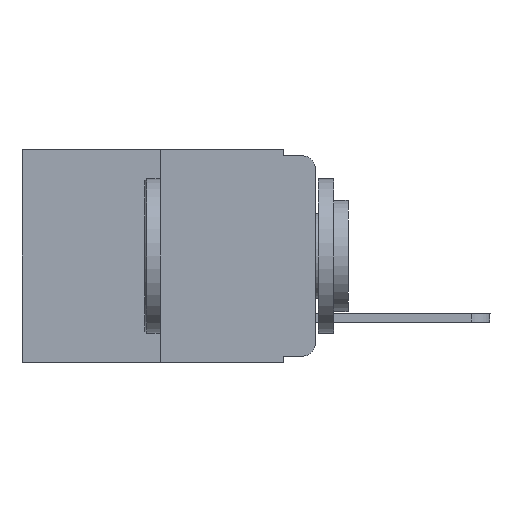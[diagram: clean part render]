
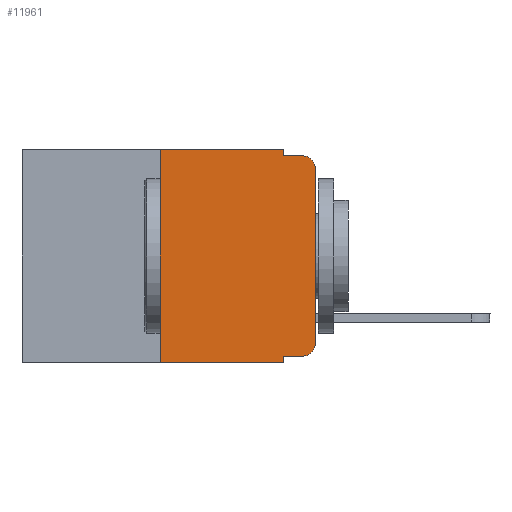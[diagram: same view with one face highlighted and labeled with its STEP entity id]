
A CAD part, left-side view. The second image highlights one B-rep face of the part: STEP entity #11961.
In plain terms, the highlighted planar face has unit normal (-1, 0, 0).
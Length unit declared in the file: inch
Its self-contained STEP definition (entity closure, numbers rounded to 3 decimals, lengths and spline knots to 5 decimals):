
#108 = CARTESIAN_POINT ( 'NONE',  ( 0., 0.02, -0.03 ) ) ;
#136 = DIRECTION ( 'NONE',  ( 0., 0., 1. ) ) ;
#485 = EDGE_CURVE ( 'NONE', #8665, #13076, #2736, .T. ) ;
#752 = VECTOR ( 'NONE', #2360, 39.37008 ) ;
#754 = ORIENTED_EDGE ( 'NONE', *, *, #22057, .T. ) ;
#1009 = DIRECTION ( 'NONE',  ( -1., 0., 0. ) ) ;
#1392 = CIRCLE ( 'NONE', #2554, 0.02 ) ;
#1819 = EDGE_CURVE ( 'NONE', #18879, #10111, #19831, .T. ) ;
#2360 = DIRECTION ( 'NONE',  ( 0., 0., -1. ) ) ;
#2554 = AXIS2_PLACEMENT_3D ( 'NONE', #108, #14737, #12557 ) ;
#2681 = CARTESIAN_POINT ( 'NONE',  ( 0., 0.473, 0. ) ) ;
#2736 = CIRCLE ( 'NONE', #9696, 0.02 ) ;
#2894 = DIRECTION ( 'NONE',  ( 0., -1., 0. ) ) ;
#3457 = ORIENTED_EDGE ( 'NONE', *, *, #5356, .F. ) ;
#3514 = VERTEX_POINT ( 'NONE', #14133 ) ;
#3524 = LINE ( 'NONE', #22312, #7562 ) ;
#3659 = VECTOR ( 'NONE', #22688, 39.37008 ) ;
#3945 = LINE ( 'NONE', #9612, #752 ) ;
#3981 = LINE ( 'NONE', #17259, #8720 ) ;
#4107 = VERTEX_POINT ( 'NONE', #16876 ) ;
#4169 = ORIENTED_EDGE ( 'NONE', *, *, #1819, .F. ) ;
#5329 = DIRECTION ( 'NONE',  ( 1., 0., 0. ) ) ;
#5356 = EDGE_CURVE ( 'NONE', #3514, #12157, #3945, .T. ) ;
#5535 = EDGE_CURVE ( 'NONE', #13076, #16201, #22835, .T. ) ;
#5850 = VECTOR ( 'NONE', #2894, 39.37008 ) ;
#6063 = VECTOR ( 'NONE', #17531, 39.37008 ) ;
#6206 = EDGE_CURVE ( 'NONE', #23818, #17589, #3524, .T. ) ;
#6356 = ORIENTED_EDGE ( 'NONE', *, *, #6206, .F. ) ;
#6937 = DIRECTION ( 'NONE',  ( 0., 0., -1. ) ) ;
#7132 = ORIENTED_EDGE ( 'NONE', *, *, #15528, .F. ) ;
#7562 = VECTOR ( 'NONE', #136, 39.37008 ) ;
#7708 = CARTESIAN_POINT ( 'NONE',  ( 0., 0., -0.03 ) ) ;
#7861 = CARTESIAN_POINT ( 'NONE',  ( 0., 0.051, -0.343 ) ) ;
#8154 = CARTESIAN_POINT ( 'NONE',  ( 0., 0., 0. ) ) ;
#8665 = VERTEX_POINT ( 'NONE', #22729 ) ;
#8720 = VECTOR ( 'NONE', #22639, 39.37008 ) ;
#8829 = FACE_OUTER_BOUND ( 'NONE', #22675, .T. ) ;
#8880 = ORIENTED_EDGE ( 'NONE', *, *, #5535, .T. ) ;
#9612 = CARTESIAN_POINT ( 'NONE',  ( 0., 0.051, 0. ) ) ;
#9696 = AXIS2_PLACEMENT_3D ( 'NONE', #21606, #1009, #10321 ) ;
#10111 = VERTEX_POINT ( 'NONE', #16545 ) ;
#10147 = LINE ( 'NONE', #12314, #5850 ) ;
#10174 = LINE ( 'NONE', #2681, #6063 ) ;
#10321 = DIRECTION ( 'NONE',  ( 0., 0., -1. ) ) ;
#10391 = CARTESIAN_POINT ( 'NONE',  ( 0., 0.25, -0.343 ) ) ;
#10906 = ORIENTED_EDGE ( 'NONE', *, *, #485, .T. ) ;
#11953 = AXIS2_PLACEMENT_3D ( 'NONE', #18220, #5329, #15962 ) ;
#11961 = ADVANCED_FACE ( 'NONE', ( #8829 ), #23626, .F. ) ;
#12058 = VECTOR ( 'NONE', #6937, 39.37008 ) ;
#12157 = VERTEX_POINT ( 'NONE', #7861 ) ;
#12314 = CARTESIAN_POINT ( 'NONE',  ( 0., 0.051, -0.01 ) ) ;
#12557 = DIRECTION ( 'NONE',  ( 0., 0., -1. ) ) ;
#13076 = VERTEX_POINT ( 'NONE', #23027 ) ;
#13822 = ORIENTED_EDGE ( 'NONE', *, *, #21860, .T. ) ;
#14133 = CARTESIAN_POINT ( 'NONE',  ( 0., 0.051, -0.333 ) ) ;
#14737 = DIRECTION ( 'NONE',  ( -1., 0., 0. ) ) ;
#15136 = LINE ( 'NONE', #15371, #3659 ) ;
#15185 = ORIENTED_EDGE ( 'NONE', *, *, #22885, .F. ) ;
#15371 = CARTESIAN_POINT ( 'NONE',  ( 0., 0.473, -0.343 ) ) ;
#15528 = EDGE_CURVE ( 'NONE', #10111, #4107, #10147, .T. ) ;
#15962 = DIRECTION ( 'NONE',  ( 0., 0., -1. ) ) ;
#16201 = VERTEX_POINT ( 'NONE', #7708 ) ;
#16545 = CARTESIAN_POINT ( 'NONE',  ( 0., 0.051, -0.01 ) ) ;
#16876 = CARTESIAN_POINT ( 'NONE',  ( 0., 0.02, -0.01 ) ) ;
#16978 = VECTOR ( 'NONE', #21252, 39.37008 ) ;
#17259 = CARTESIAN_POINT ( 'NONE',  ( 0., 0.051, -0.333 ) ) ;
#17531 = DIRECTION ( 'NONE',  ( 0., -1., 0. ) ) ;
#17589 = VERTEX_POINT ( 'NONE', #20920 ) ;
#18220 = CARTESIAN_POINT ( 'NONE',  ( 0., 0.473, 0. ) ) ;
#18879 = VERTEX_POINT ( 'NONE', #21982 ) ;
#19598 = CARTESIAN_POINT ( 'NONE',  ( 0., 0.051, 0. ) ) ;
#19831 = LINE ( 'NONE', #19598, #12058 ) ;
#20011 = EDGE_CURVE ( 'NONE', #23818, #12157, #15136, .T. ) ;
#20920 = CARTESIAN_POINT ( 'NONE',  ( 0., 0.25, 0. ) ) ;
#21252 = DIRECTION ( 'NONE',  ( 0., 0., 1. ) ) ;
#21606 = CARTESIAN_POINT ( 'NONE',  ( 0., 0.02, -0.313 ) ) ;
#21860 = EDGE_CURVE ( 'NONE', #16201, #4107, #1392, .T. ) ;
#21982 = CARTESIAN_POINT ( 'NONE',  ( 0., 0.051, 0. ) ) ;
#22057 = EDGE_CURVE ( 'NONE', #3514, #8665, #3981, .T. ) ;
#22312 = CARTESIAN_POINT ( 'NONE',  ( 0., 0.25, 0. ) ) ;
#22639 = DIRECTION ( 'NONE',  ( 0., -1., 0. ) ) ;
#22675 = EDGE_LOOP ( 'NONE', ( #8880, #13822, #7132, #4169, #15185, #6356, #23849, #3457, #754, #10906 ) ) ;
#22688 = DIRECTION ( 'NONE',  ( 0., -1., 0. ) ) ;
#22729 = CARTESIAN_POINT ( 'NONE',  ( 0., 0.02, -0.333 ) ) ;
#22835 = LINE ( 'NONE', #8154, #16978 ) ;
#22885 = EDGE_CURVE ( 'NONE', #17589, #18879, #10174, .T. ) ;
#23027 = CARTESIAN_POINT ( 'NONE',  ( 0., 0., -0.313 ) ) ;
#23626 = PLANE ( 'NONE',  #11953 ) ;
#23818 = VERTEX_POINT ( 'NONE', #10391 ) ;
#23849 = ORIENTED_EDGE ( 'NONE', *, *, #20011, .T. ) ;
